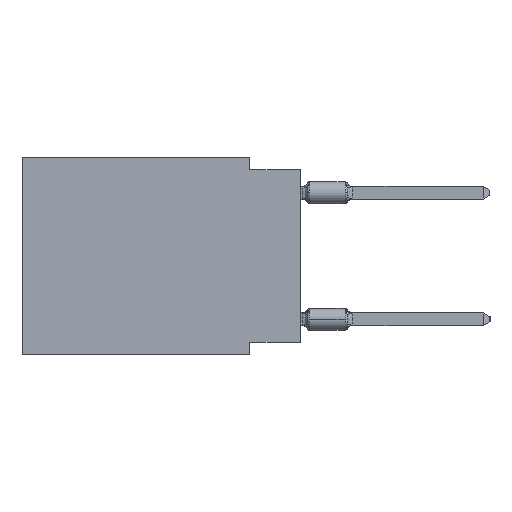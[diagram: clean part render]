
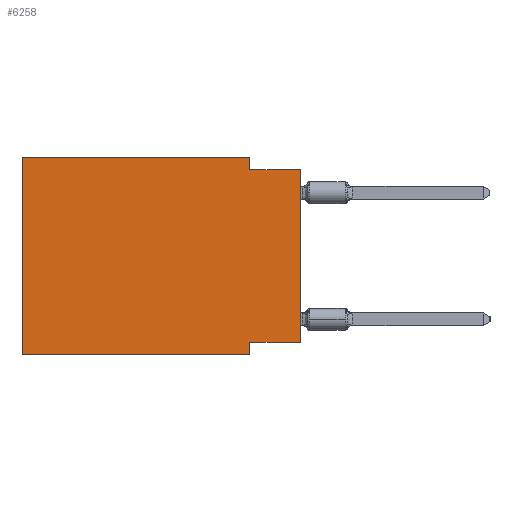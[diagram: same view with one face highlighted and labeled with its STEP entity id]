
A CAD part, left-side view. The second image highlights one B-rep face of the part: STEP entity #6258.
In plain terms, the highlighted planar face has unit normal (-1, 0, 0).
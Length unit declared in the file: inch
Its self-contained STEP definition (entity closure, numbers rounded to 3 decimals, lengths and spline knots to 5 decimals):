
#95 = VECTOR ( 'NONE', #9771, 39.37008 ) ;
#196 = LINE ( 'NONE', #20643, #11839 ) ;
#754 = CARTESIAN_POINT ( 'NONE',  ( 0., 0.55, 0. ) ) ;
#902 = LINE ( 'NONE', #8604, #22875 ) ;
#1138 = VERTEX_POINT ( 'NONE', #15843 ) ;
#1387 = DIRECTION ( 'NONE',  ( 0., -1., 0. ) ) ;
#2105 = EDGE_CURVE ( 'NONE', #2297, #16461, #12006, .T. ) ;
#2229 = DIRECTION ( 'NONE',  ( 0., 0., 1. ) ) ;
#2297 = VERTEX_POINT ( 'NONE', #22311 ) ;
#2315 = LINE ( 'NONE', #20935, #95 ) ;
#3424 = CARTESIAN_POINT ( 'NONE',  ( 0., 0.55, 0. ) ) ;
#3448 = ORIENTED_EDGE ( 'NONE', *, *, #6988, .F. ) ;
#3511 = VERTEX_POINT ( 'NONE', #20614 ) ;
#3705 = DIRECTION ( 'NONE',  ( 1., 0., 0. ) ) ;
#3728 = VECTOR ( 'NONE', #19763, 39.37008 ) ;
#3797 = DIRECTION ( 'NONE',  ( 0., -1., 0. ) ) ;
#4106 = DIRECTION ( 'NONE',  ( 0., 0., -1. ) ) ;
#4414 = LINE ( 'NONE', #23128, #10524 ) ;
#5142 = EDGE_CURVE ( 'NONE', #17461, #1138, #4414, .T. ) ;
#5445 = AXIS2_PLACEMENT_3D ( 'NONE', #18508, #3705, #9320 ) ;
#5524 = ORIENTED_EDGE ( 'NONE', *, *, #24006, .T. ) ;
#6258 = ADVANCED_FACE ( 'NONE', ( #13674 ), #11019, .F. ) ;
#6398 = ORIENTED_EDGE ( 'NONE', *, *, #2105, .F. ) ;
#6477 = DIRECTION ( 'NONE',  ( 0., 1., 0. ) ) ;
#6988 = EDGE_CURVE ( 'NONE', #1138, #19492, #16939, .T. ) ;
#7077 = LINE ( 'NONE', #3424, #12272 ) ;
#8604 = CARTESIAN_POINT ( 'NONE',  ( 0., 0.55, -0.39 ) ) ;
#9320 = DIRECTION ( 'NONE',  ( 0., 0., -1. ) ) ;
#9600 = EDGE_LOOP ( 'NONE', ( #5524, #15528, #11387, #23886, #6398, #15390, #3448, #20176 ) ) ;
#9771 = DIRECTION ( 'NONE',  ( 0., -1., 0. ) ) ;
#10060 = CARTESIAN_POINT ( 'NONE',  ( 0., 0., -0.365 ) ) ;
#10197 = CARTESIAN_POINT ( 'NONE',  ( 0., 0., 0. ) ) ;
#10524 = VECTOR ( 'NONE', #6477, 39.37008 ) ;
#11019 = PLANE ( 'NONE',  #5445 ) ;
#11387 = ORIENTED_EDGE ( 'NONE', *, *, #12201, .F. ) ;
#11639 = EDGE_CURVE ( 'NONE', #16461, #3511, #7077, .T. ) ;
#11747 = CARTESIAN_POINT ( 'NONE',  ( 0., 0.1, -0.025 ) ) ;
#11839 = VECTOR ( 'NONE', #18798, 39.37008 ) ;
#12006 = LINE ( 'NONE', #754, #17105 ) ;
#12201 = EDGE_CURVE ( 'NONE', #3511, #13200, #196, .T. ) ;
#12272 = VECTOR ( 'NONE', #3797, 39.37008 ) ;
#13200 = VERTEX_POINT ( 'NONE', #11747 ) ;
#13674 = FACE_OUTER_BOUND ( 'NONE', #9600, .T. ) ;
#15029 = EDGE_CURVE ( 'NONE', #13200, #16509, #2315, .T. ) ;
#15062 = CARTESIAN_POINT ( 'NONE',  ( 0., 0., -0.025 ) ) ;
#15390 = ORIENTED_EDGE ( 'NONE', *, *, #23899, .T. ) ;
#15528 = ORIENTED_EDGE ( 'NONE', *, *, #15029, .F. ) ;
#15743 = CARTESIAN_POINT ( 'NONE',  ( 0., 0.1, -0.39 ) ) ;
#15843 = CARTESIAN_POINT ( 'NONE',  ( 0., 0.1, -0.365 ) ) ;
#16461 = VERTEX_POINT ( 'NONE', #18122 ) ;
#16509 = VERTEX_POINT ( 'NONE', #15062 ) ;
#16939 = LINE ( 'NONE', #20873, #21886 ) ;
#17105 = VECTOR ( 'NONE', #2229, 39.37008 ) ;
#17461 = VERTEX_POINT ( 'NONE', #10060 ) ;
#18122 = CARTESIAN_POINT ( 'NONE',  ( 0., 0.55, 0. ) ) ;
#18155 = LINE ( 'NONE', #10197, #3728 ) ;
#18508 = CARTESIAN_POINT ( 'NONE',  ( 0., 0.55, 0. ) ) ;
#18798 = DIRECTION ( 'NONE',  ( 0., 0., -1. ) ) ;
#19492 = VERTEX_POINT ( 'NONE', #15743 ) ;
#19763 = DIRECTION ( 'NONE',  ( 0., 0., 1. ) ) ;
#20176 = ORIENTED_EDGE ( 'NONE', *, *, #5142, .F. ) ;
#20614 = CARTESIAN_POINT ( 'NONE',  ( 0., 0.1, 0. ) ) ;
#20643 = CARTESIAN_POINT ( 'NONE',  ( 0., 0.1, 0. ) ) ;
#20873 = CARTESIAN_POINT ( 'NONE',  ( 0., 0.1, -0.39 ) ) ;
#20935 = CARTESIAN_POINT ( 'NONE',  ( 0., 0., -0.025 ) ) ;
#21886 = VECTOR ( 'NONE', #4106, 39.37008 ) ;
#22311 = CARTESIAN_POINT ( 'NONE',  ( 0., 0.55, -0.39 ) ) ;
#22875 = VECTOR ( 'NONE', #1387, 39.37008 ) ;
#23128 = CARTESIAN_POINT ( 'NONE',  ( 0., 0., -0.365 ) ) ;
#23886 = ORIENTED_EDGE ( 'NONE', *, *, #11639, .F. ) ;
#23899 = EDGE_CURVE ( 'NONE', #2297, #19492, #902, .T. ) ;
#24006 = EDGE_CURVE ( 'NONE', #17461, #16509, #18155, .T. ) ;
